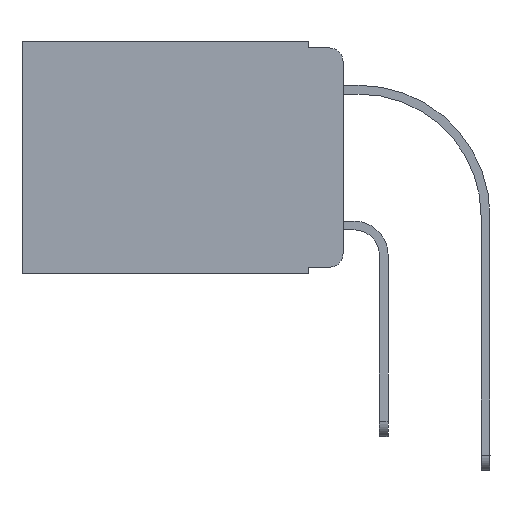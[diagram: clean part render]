
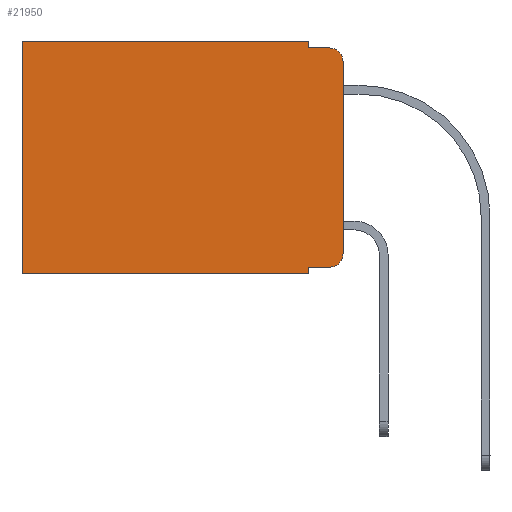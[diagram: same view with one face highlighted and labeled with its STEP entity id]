
A CAD part, left-side view. The second image highlights one B-rep face of the part: STEP entity #21950.
In plain terms, the highlighted planar face has unit normal (-1, 0, 0).
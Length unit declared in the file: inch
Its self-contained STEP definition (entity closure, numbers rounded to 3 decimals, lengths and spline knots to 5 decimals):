
#67 = CARTESIAN_POINT ( 'NONE',  ( 0.298, 0., -0.313 ) ) ;
#343 = EDGE_CURVE ( 'NONE', #25047, #14148, #10378, .T. ) ;
#363 = CARTESIAN_POINT ( 'NONE',  ( 0.298, 0.02, -0.333 ) ) ;
#373 = CARTESIAN_POINT ( 'NONE',  ( 0.298, 0.473, 0. ) ) ;
#634 = DIRECTION ( 'NONE',  ( 1., 0., 0. ) ) ;
#1559 = LINE ( 'NONE', #9805, #24300 ) ;
#1847 = CARTESIAN_POINT ( 'NONE',  ( 0.298, 0.473, -0.343 ) ) ;
#1867 = LINE ( 'NONE', #3664, #16390 ) ;
#1966 = EDGE_CURVE ( 'NONE', #11414, #13430, #16831, .T. ) ;
#2191 = DIRECTION ( 'NONE',  ( -1., 0., 0. ) ) ;
#2502 = CARTESIAN_POINT ( 'NONE',  ( 0.298, 0.473, 0. ) ) ;
#2507 = DIRECTION ( 'NONE',  ( 0., -1., 0. ) ) ;
#3366 = DIRECTION ( 'NONE',  ( 0., 0., -1. ) ) ;
#3664 = CARTESIAN_POINT ( 'NONE',  ( 0.298, 0., -0.343 ) ) ;
#3960 = VECTOR ( 'NONE', #22527, 39.37008 ) ;
#4117 = DIRECTION ( 'NONE',  ( 0., 0., -1. ) ) ;
#4161 = DIRECTION ( 'NONE',  ( 0., 1., 0. ) ) ;
#4167 = ORIENTED_EDGE ( 'NONE', *, *, #343, .T. ) ;
#4448 = CARTESIAN_POINT ( 'NONE',  ( 0.298, 0.051, -0.333 ) ) ;
#4687 = CARTESIAN_POINT ( 'NONE',  ( 0.298, 0., 0. ) ) ;
#4787 = VERTEX_POINT ( 'NONE', #1847 ) ;
#5452 = AXIS2_PLACEMENT_3D ( 'NONE', #17083, #24953, #3366 ) ;
#5778 = CARTESIAN_POINT ( 'NONE',  ( 0.298, 0., 0. ) ) ;
#6059 = CARTESIAN_POINT ( 'NONE',  ( 0.298, 0.02, -0.313 ) ) ;
#6201 = CIRCLE ( 'NONE', #5452, 0.02 ) ;
#6472 = EDGE_CURVE ( 'NONE', #23608, #14148, #15719, .T. ) ;
#7513 = VERTEX_POINT ( 'NONE', #8537 ) ;
#7624 = VERTEX_POINT ( 'NONE', #13066 ) ;
#7665 = LINE ( 'NONE', #13603, #15922 ) ;
#7743 = DIRECTION ( 'NONE',  ( 0., 0., -1. ) ) ;
#7789 = DIRECTION ( 'NONE',  ( 0., 0., -1. ) ) ;
#7799 = EDGE_CURVE ( 'NONE', #11414, #7624, #1559, .T. ) ;
#8074 = ORIENTED_EDGE ( 'NONE', *, *, #17053, .T. ) ;
#8537 = CARTESIAN_POINT ( 'NONE',  ( 0.298, 0.02, -0.01 ) ) ;
#9805 = CARTESIAN_POINT ( 'NONE',  ( 0.298, 0.051, 0. ) ) ;
#10067 = PLANE ( 'NONE',  #16624 ) ;
#10305 = LINE ( 'NONE', #12381, #11016 ) ;
#10378 = CIRCLE ( 'NONE', #12872, 0.02 ) ;
#10452 = FACE_OUTER_BOUND ( 'NONE', #17021, .T. ) ;
#10518 = LINE ( 'NONE', #4448, #15972 ) ;
#11016 = VECTOR ( 'NONE', #20260, 39.37008 ) ;
#11251 = CARTESIAN_POINT ( 'NONE',  ( 0.298, 0.051, 0. ) ) ;
#11414 = VERTEX_POINT ( 'NONE', #11251 ) ;
#11544 = EDGE_CURVE ( 'NONE', #7624, #7513, #10305, .T. ) ;
#11961 = DIRECTION ( 'NONE',  ( 0., 0., -1. ) ) ;
#12381 = CARTESIAN_POINT ( 'NONE',  ( 0.298, 0.051, -0.01 ) ) ;
#12872 = AXIS2_PLACEMENT_3D ( 'NONE', #6059, #2191, #7743 ) ;
#13066 = CARTESIAN_POINT ( 'NONE',  ( 0.298, 0.051, -0.01 ) ) ;
#13196 = EDGE_CURVE ( 'NONE', #23608, #7513, #6201, .T. ) ;
#13360 = ORIENTED_EDGE ( 'NONE', *, *, #16019, .F. ) ;
#13430 = VERTEX_POINT ( 'NONE', #373 ) ;
#13603 = CARTESIAN_POINT ( 'NONE',  ( 0.298, 0.051, 0. ) ) ;
#13663 = ORIENTED_EDGE ( 'NONE', *, *, #1966, .T. ) ;
#14148 = VERTEX_POINT ( 'NONE', #67 ) ;
#14812 = CARTESIAN_POINT ( 'NONE',  ( 0.298, 0.051, -0.343 ) ) ;
#15620 = CARTESIAN_POINT ( 'NONE',  ( 0.298, 0., -0.03 ) ) ;
#15643 = ORIENTED_EDGE ( 'NONE', *, *, #18506, .T. ) ;
#15719 = LINE ( 'NONE', #5778, #20986 ) ;
#15922 = VECTOR ( 'NONE', #7789, 39.37008 ) ;
#15972 = VECTOR ( 'NONE', #2507, 39.37008 ) ;
#16019 = EDGE_CURVE ( 'NONE', #19821, #22586, #7665, .T. ) ;
#16390 = VECTOR ( 'NONE', #4161, 39.37008 ) ;
#16504 = ORIENTED_EDGE ( 'NONE', *, *, #17302, .F. ) ;
#16624 = AXIS2_PLACEMENT_3D ( 'NONE', #18338, #634, #4117 ) ;
#16831 = LINE ( 'NONE', #4687, #23834 ) ;
#17021 = EDGE_LOOP ( 'NONE', ( #19388, #18864, #22417, #17734, #13663, #15643, #16504, #13360, #8074, #4167 ) ) ;
#17053 = EDGE_CURVE ( 'NONE', #19821, #25047, #10518, .T. ) ;
#17083 = CARTESIAN_POINT ( 'NONE',  ( 0.298, 0.02, -0.03 ) ) ;
#17302 = EDGE_CURVE ( 'NONE', #22586, #4787, #1867, .T. ) ;
#17734 = ORIENTED_EDGE ( 'NONE', *, *, #7799, .F. ) ;
#18338 = CARTESIAN_POINT ( 'NONE',  ( 0.298, 0., 0. ) ) ;
#18506 = EDGE_CURVE ( 'NONE', #13430, #4787, #20204, .T. ) ;
#18864 = ORIENTED_EDGE ( 'NONE', *, *, #13196, .T. ) ;
#19250 = DIRECTION ( 'NONE',  ( 0., 0., -1. ) ) ;
#19388 = ORIENTED_EDGE ( 'NONE', *, *, #6472, .F. ) ;
#19821 = VERTEX_POINT ( 'NONE', #24242 ) ;
#20204 = LINE ( 'NONE', #2502, #3960 ) ;
#20260 = DIRECTION ( 'NONE',  ( 0., -1., 0. ) ) ;
#20986 = VECTOR ( 'NONE', #11961, 39.37008 ) ;
#21950 = ADVANCED_FACE ( 'NONE', ( #10452 ), #10067, .F. ) ;
#22417 = ORIENTED_EDGE ( 'NONE', *, *, #11544, .F. ) ;
#22527 = DIRECTION ( 'NONE',  ( 0., 0., -1. ) ) ;
#22586 = VERTEX_POINT ( 'NONE', #14812 ) ;
#23608 = VERTEX_POINT ( 'NONE', #15620 ) ;
#23834 = VECTOR ( 'NONE', #24303, 39.37008 ) ;
#24242 = CARTESIAN_POINT ( 'NONE',  ( 0.298, 0.051, -0.333 ) ) ;
#24300 = VECTOR ( 'NONE', #19250, 39.37008 ) ;
#24303 = DIRECTION ( 'NONE',  ( 0., 1., 0. ) ) ;
#24953 = DIRECTION ( 'NONE',  ( -1., 0., 0. ) ) ;
#25047 = VERTEX_POINT ( 'NONE', #363 ) ;
